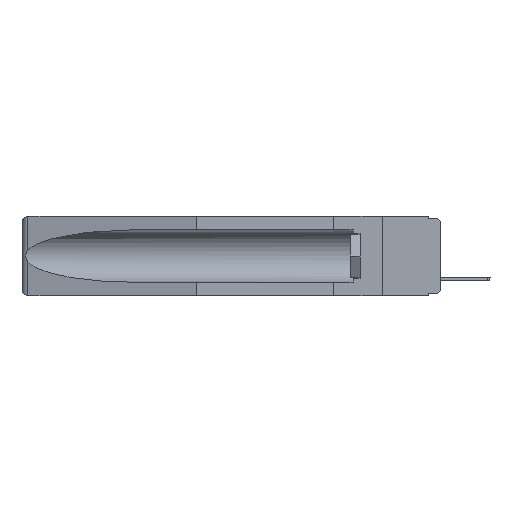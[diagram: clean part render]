
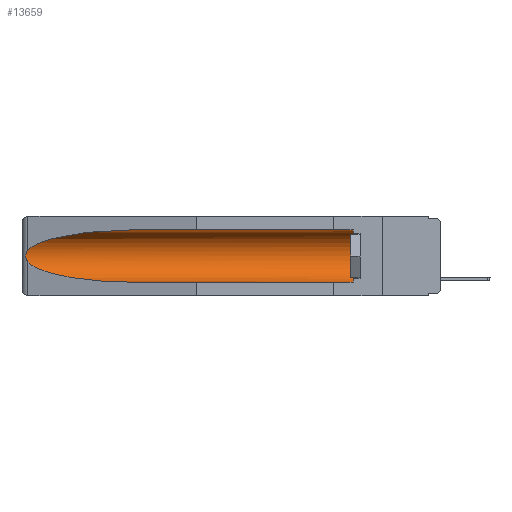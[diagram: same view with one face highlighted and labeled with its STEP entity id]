
A CAD part, left-side view. The second image highlights one B-rep face of the part: STEP entity #13659.
In plain terms, the highlighted cylindrical face has radius 2.857 mm (diameter 5.715 mm), a partial arc.
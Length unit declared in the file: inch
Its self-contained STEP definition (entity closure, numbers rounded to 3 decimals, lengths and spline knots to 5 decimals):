
#151 = ORIENTED_EDGE ( 'NONE', *, *, #15410, .T. ) ;
#674 = CYLINDRICAL_SURFACE ( 'NONE', #13661, 0.1125 ) ;
#1210 = LINE ( 'NONE', #11054, #18464 ) ;
#1967 =( BOUNDED_CURVE ( )  B_SPLINE_CURVE ( 3, ( #3595, #9775, #9902, #7934 ),
 .UNSPECIFIED., .F., .F. ) 
 B_SPLINE_CURVE_WITH_KNOTS ( ( 4, 4 ),
 ( 0.1948, 1.5708 ),
 .UNSPECIFIED. ) 
 CURVE ( )  GEOMETRIC_REPRESENTATION_ITEM ( )  RATIONAL_B_SPLINE_CURVE ( ( 1., 0.848, 0.848, 1. ) ) 
 REPRESENTATION_ITEM ( '' )  );
#2910 = EDGE_CURVE ( 'NONE', #4809, #18221, #1210, .T. ) ;
#3040 = DIRECTION ( 'NONE',  ( 0., 1., 0. ) ) ;
#3173 = FACE_OUTER_BOUND ( 'NONE', #10962, .T. ) ;
#3595 = CARTESIAN_POINT ( 'NONE',  ( 0.26537, 1.52718, -0.19328 ) ) ;
#3901 = CARTESIAN_POINT ( 'NONE',  ( 0.155, -0.30754, -0.059 ) ) ;
#4348 = CARTESIAN_POINT ( 'NONE',  ( 0.25451, 1.48313, -0.09465 ) ) ;
#4809 = VERTEX_POINT ( 'NONE', #22279 ) ;
#5390 = ORIENTED_EDGE ( 'NONE', *, *, #12535, .T. ) ;
#6072 = CARTESIAN_POINT ( 'NONE',  ( 0.21114, 1.30732, -0.059 ) ) ;
#6260 = CARTESIAN_POINT ( 'NONE',  ( 0.26597, 1.52961, -0.15275 ) ) ;
#6514 = CARTESIAN_POINT ( 'NONE',  ( 0.2675, 1.53308, -0.16763 ) ) ;
#6656 = CARTESIAN_POINT ( 'NONE',  ( 0.26654, 1.53092, -0.15636 ) ) ;
#6980 = ORIENTED_EDGE ( 'NONE', *, *, #2910, .F. ) ;
#7055 = VERTEX_POINT ( 'NONE', #22124 ) ;
#7934 = CARTESIAN_POINT ( 'NONE',  ( 0.155, 1.07973, -0.284 ) ) ;
#8641 = CARTESIAN_POINT ( 'NONE',  ( 0.26537, 1.52718, -0.14972 ) ) ;
#8704 = CARTESIAN_POINT ( 'NONE',  ( 0.155, -0.30754, -0.1715 ) ) ;
#8852 = ORIENTED_EDGE ( 'NONE', *, *, #14576, .T. ) ;
#9559 = VECTOR ( 'NONE', #19794, 39.37008 ) ;
#9775 = CARTESIAN_POINT ( 'NONE',  ( 0.25451, 1.48313, -0.24835 ) ) ;
#9902 = CARTESIAN_POINT ( 'NONE',  ( 0.21114, 1.30732, -0.284 ) ) ;
#9958 = LINE ( 'NONE', #3901, #9559 ) ;
#10799 = VERTEX_POINT ( 'NONE', #13139 ) ;
#10821 = CARTESIAN_POINT ( 'NONE',  ( 0.155, 0.126, -0.1715 ) ) ;
#10870 = CARTESIAN_POINT ( 'NONE',  ( 0.2673, 1.5327, -0.16383 ) ) ;
#10962 = EDGE_LOOP ( 'NONE', ( #151, #8852, #25214, #6980, #22513, #5390 ) ) ;
#11054 = CARTESIAN_POINT ( 'NONE',  ( 0.155, -0.30754, -0.284 ) ) ;
#11208 = CARTESIAN_POINT ( 'NONE',  ( 0.155, 1.07973, -0.284 ) ) ;
#12535 = EDGE_CURVE ( 'NONE', #10799, #14652, #9958, .T. ) ;
#12562 = CARTESIAN_POINT ( 'NONE',  ( 0.2675, 1.53308, -0.17534 ) ) ;
#12829 = CARTESIAN_POINT ( 'NONE',  ( 0.26655, 1.53094, -0.18657 ) ) ;
#13139 = CARTESIAN_POINT ( 'NONE',  ( 0.155, 0.126, -0.059 ) ) ;
#13659 = ADVANCED_FACE ( 'NONE', ( #3173 ), #674, .F. ) ;
#13661 = AXIS2_PLACEMENT_3D ( 'NONE', #8704, #3040, #16690 ) ;
#14462 = CARTESIAN_POINT ( 'NONE',  ( 0.155, 1.07973, -0.059 ) ) ;
#14576 = EDGE_CURVE ( 'NONE', #16140, #7055, #21983, .T. ) ;
#14652 = VERTEX_POINT ( 'NONE', #25305 ) ;
#15300 = EDGE_CURVE ( 'NONE', #7055, #18221, #1967, .T. ) ;
#15410 = EDGE_CURVE ( 'NONE', #14652, #16140, #19912, .T. ) ;
#15925 = AXIS2_PLACEMENT_3D ( 'NONE', #10821, #22233, #18539 ) ;
#16140 = VERTEX_POINT ( 'NONE', #23587 ) ;
#16690 = DIRECTION ( 'NONE',  ( 0., 0., 1. ) ) ;
#17190 = CIRCLE ( 'NONE', #15925, 0.1125 ) ;
#18135 = CARTESIAN_POINT ( 'NONE',  ( 0.26537, 1.52718, -0.14972 ) ) ;
#18154 = EDGE_CURVE ( 'NONE', #4809, #10799, #17190, .T. ) ;
#18221 = VERTEX_POINT ( 'NONE', #11208 ) ;
#18464 = VECTOR ( 'NONE', #25109, 39.37008 ) ;
#18539 = DIRECTION ( 'NONE',  ( 0., 0., 1. ) ) ;
#18729 = CARTESIAN_POINT ( 'NONE',  ( 0.2673, 1.53269, -0.17917 ) ) ;
#19794 = DIRECTION ( 'NONE',  ( 0., 1., 0. ) ) ;
#19912 =( BOUNDED_CURVE ( )  B_SPLINE_CURVE ( 3, ( #14462, #6072, #4348, #18135 ),
 .UNSPECIFIED., .F., .F. ) 
 B_SPLINE_CURVE_WITH_KNOTS ( ( 4, 4 ),
 ( 4.71239, 6.08839 ),
 .UNSPECIFIED. ) 
 CURVE ( )  GEOMETRIC_REPRESENTATION_ITEM ( )  RATIONAL_B_SPLINE_CURVE ( ( 1., 0.848, 0.848, 1. ) ) 
 REPRESENTATION_ITEM ( '' )  );
#20561 = CARTESIAN_POINT ( 'NONE',  ( 0.26537, 1.52718, -0.19328 ) ) ;
#21983 = B_SPLINE_CURVE_WITH_KNOTS ( 'NONE', 3,
 ( #8641, #6260, #6656, #10870, #6514, #12562, #18729, #12829, #24642, #20561 ),
 .UNSPECIFIED., .F., .F.,
 ( 4, 2, 2, 2, 4 ),
 ( 0., 0.00029, 0.00058, 0.00087, 0.00117 ),
 .UNSPECIFIED. ) ;
#22124 = CARTESIAN_POINT ( 'NONE',  ( 0.26537, 1.52718, -0.19328 ) ) ;
#22233 = DIRECTION ( 'NONE',  ( 0., -1., 0. ) ) ;
#22279 = CARTESIAN_POINT ( 'NONE',  ( 0.155, 0.126, -0.284 ) ) ;
#22513 = ORIENTED_EDGE ( 'NONE', *, *, #18154, .T. ) ;
#23587 = CARTESIAN_POINT ( 'NONE',  ( 0.26537, 1.52718, -0.14972 ) ) ;
#24642 = CARTESIAN_POINT ( 'NONE',  ( 0.26597, 1.5296, -0.19026 ) ) ;
#25109 = DIRECTION ( 'NONE',  ( 0., 1., 0. ) ) ;
#25214 = ORIENTED_EDGE ( 'NONE', *, *, #15300, .T. ) ;
#25305 = CARTESIAN_POINT ( 'NONE',  ( 0.155, 1.07973, -0.059 ) ) ;
